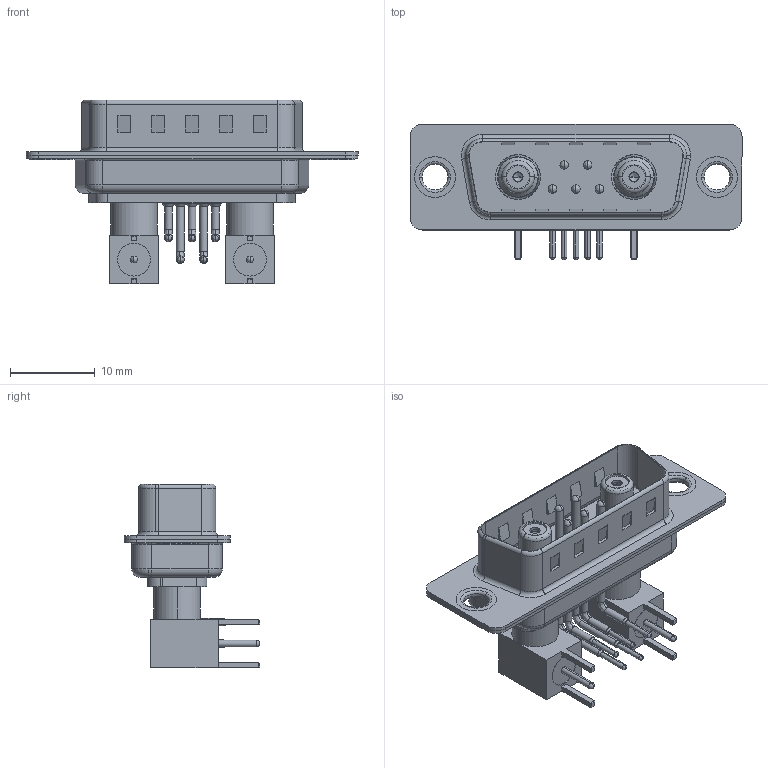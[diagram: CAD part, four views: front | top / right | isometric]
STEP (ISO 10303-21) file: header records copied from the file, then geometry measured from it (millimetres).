
FILE_DESCRIPTION (( 'STEP AP203' ), '1' );
FILE_NAME ('629-7W2-640-7N1.STEP', '2022-05-06T17:49:23', ( '' ), ( '' ), 'SwSTEP 2.0', 'SolidWorks 2020', '' );
FILE_SCHEMA (( 'CONFIG_CONTROL_DESIGN' ));
Length unit declared in the file: millimetre
Products named in the file (16): Co-Ax Jack_RA PC Tail; 629Combo Shell Rear_15 Contacts; 629Combo Contact Row 1; RA Back Shell; 629Combo Housing_7W2; Socket_RA; 629Combo Contact Row 2; Co-Ax Jack Assy_RA; Locking Collar; 629-7W2-640-7N1; Insulator Socket 2; 629Combo Shell Front_15 Contacts; Insulator RA Pin; 629Combo Thru Hole Rivet; Insulator Socket
Assembly tree (26 placements, depth 3):
  629-7W2-640-7N1
    629Combo Housing_7W2
    629Combo Shell Rear_15 Contacts
    629Combo Shell Front_15 Contacts
    629Combo Thru Hole Rivet  x2
    Co-Ax Jack Assy_RA
      Co-Ax Jack_RA PC Tail
      Insulator Socket
      Insulator Socket 2
      Locking Collar
      Socket_RA
      RA Back Shell
      Insulator RA Pin
    Co-Ax Jack Assy_RA
      Co-Ax Jack_RA PC Tail
      Insulator Socket
      Insulator Socket 2
      Locking Collar
      Socket_RA
      RA Back Shell
      Insulator RA Pin
    629Combo Contact Row 1  x2
    629Combo Contact Row 2  x3
Bounding box: 39.2 x 16 x 21.71 mm (x, y, z)
Volume: 2373.5 mm3; surface area: 6637.9 mm2
Topology: 24 solids, 24 shells, 1168 faces, 3019 edges, 1922 vertices
Faces by surface type: plane 573, cylinder 431, torus 70, cone 58, bspline 32, sphere 4
Entity records: 23352 total; most frequent: CARTESIAN_POINT 4031, DIRECTION 3805, ORIENTED_EDGE 3496, EDGE_CURVE 1748, AXIS2_PLACEMENT_3D 1377, VERTEX_POINT 1119, LINE 1051, VECTOR 1051
